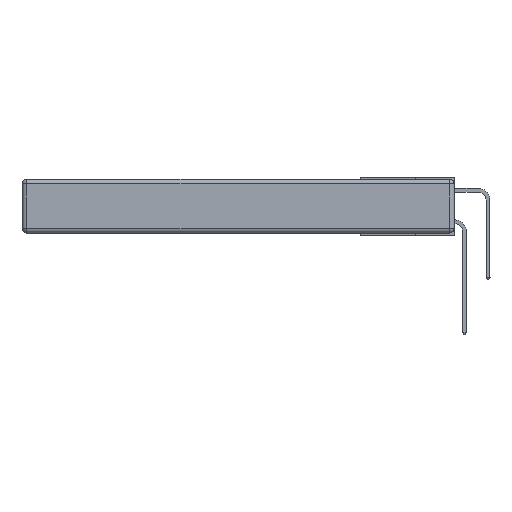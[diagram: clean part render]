
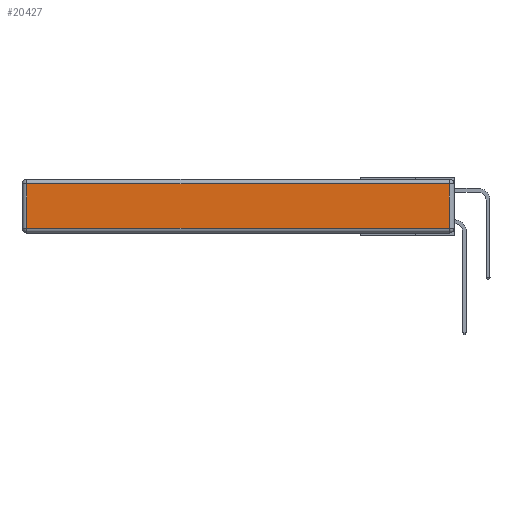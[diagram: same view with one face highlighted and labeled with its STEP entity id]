
A CAD part, left-side view. The second image highlights one B-rep face of the part: STEP entity #20427.
In plain terms, the highlighted planar face has unit normal (-1, 0, 0).
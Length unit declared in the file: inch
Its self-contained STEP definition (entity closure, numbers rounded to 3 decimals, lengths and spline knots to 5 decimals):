
#8 = ORIENTED_EDGE ( 'NONE', *, *, #4403, .T. ) ;
#1006 = ORIENTED_EDGE ( 'NONE', *, *, #21017, .T. ) ;
#1086 = LINE ( 'NONE', #7241, #25430 ) ;
#2936 = VECTOR ( 'NONE', #22970, 39.37008 ) ;
#3263 = DIRECTION ( 'NONE',  ( 0., 1., 0. ) ) ;
#4403 = EDGE_CURVE ( 'NONE', #16592, #25066, #23856, .T. ) ;
#4449 = EDGE_CURVE ( 'NONE', #24209, #16592, #1086, .T. ) ;
#5550 = CARTESIAN_POINT ( 'NONE',  ( 0., 0.03, -0.343 ) ) ;
#6089 = VECTOR ( 'NONE', #3263, 39.37008 ) ;
#7241 = CARTESIAN_POINT ( 'NONE',  ( 0., 2.72, -0.343 ) ) ;
#8197 = DIRECTION ( 'NONE',  ( 0., 0., 1. ) ) ;
#8511 = DIRECTION ( 'NONE',  ( -1., 0., 0. ) ) ;
#8594 = CARTESIAN_POINT ( 'NONE',  ( 0., 2.72, -0.313 ) ) ;
#9218 = CARTESIAN_POINT ( 'NONE',  ( 0., 0.03, -0.313 ) ) ;
#9513 = DIRECTION ( 'NONE',  ( 0., 0., -1. ) ) ;
#10795 = CARTESIAN_POINT ( 'NONE',  ( 0., 0.03, -0.03 ) ) ;
#13422 = CARTESIAN_POINT ( 'NONE',  ( 0., 2.75, -0.03 ) ) ;
#14417 = VECTOR ( 'NONE', #25014, 39.37008 ) ;
#14919 = CARTESIAN_POINT ( 'NONE',  ( 0., 0., -0.313 ) ) ;
#14993 = ORIENTED_EDGE ( 'NONE', *, *, #26980, .T. ) ;
#15119 = FACE_OUTER_BOUND ( 'NONE', #18654, .T. ) ;
#15777 = CARTESIAN_POINT ( 'NONE',  ( 0., 0., -0.343 ) ) ;
#15866 = CARTESIAN_POINT ( 'NONE',  ( 0., 2.72, -0.03 ) ) ;
#16592 = VERTEX_POINT ( 'NONE', #8594 ) ;
#18654 = EDGE_LOOP ( 'NONE', ( #8, #1006, #14993, #26795 ) ) ;
#19762 = LINE ( 'NONE', #5550, #2936 ) ;
#20427 = ADVANCED_FACE ( 'NONE', ( #15119 ), #21104, .T. ) ;
#21017 = EDGE_CURVE ( 'NONE', #25066, #25408, #19762, .T. ) ;
#21104 = PLANE ( 'NONE',  #25341 ) ;
#22970 = DIRECTION ( 'NONE',  ( 0., 0., 1. ) ) ;
#23856 = LINE ( 'NONE', #14919, #14417 ) ;
#24209 = VERTEX_POINT ( 'NONE', #15866 ) ;
#25014 = DIRECTION ( 'NONE',  ( 0., -1., 0. ) ) ;
#25066 = VERTEX_POINT ( 'NONE', #9218 ) ;
#25341 = AXIS2_PLACEMENT_3D ( 'NONE', #15777, #8511, #8197 ) ;
#25408 = VERTEX_POINT ( 'NONE', #10795 ) ;
#25430 = VECTOR ( 'NONE', #9513, 39.37008 ) ;
#26127 = LINE ( 'NONE', #13422, #6089 ) ;
#26795 = ORIENTED_EDGE ( 'NONE', *, *, #4449, .T. ) ;
#26980 = EDGE_CURVE ( 'NONE', #25408, #24209, #26127, .T. ) ;
